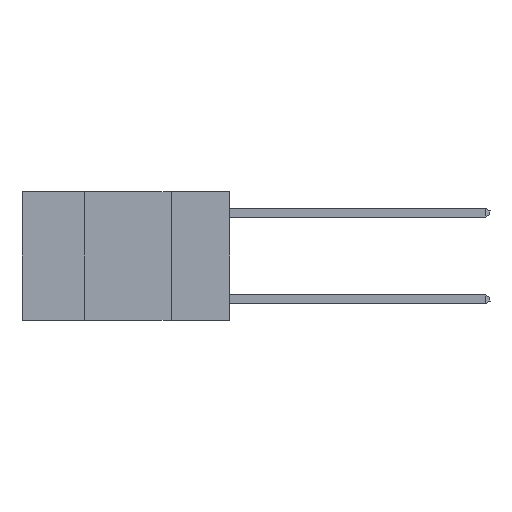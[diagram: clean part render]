
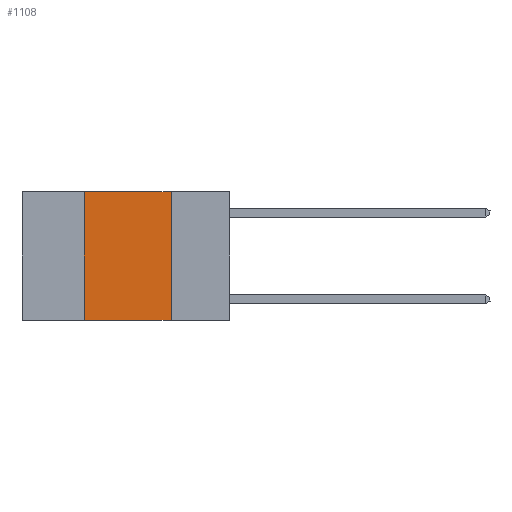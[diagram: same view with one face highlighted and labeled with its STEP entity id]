
A CAD part, left-side view. The second image highlights one B-rep face of the part: STEP entity #1108.
In plain terms, the highlighted planar face has unit normal (-1, 0, 0).
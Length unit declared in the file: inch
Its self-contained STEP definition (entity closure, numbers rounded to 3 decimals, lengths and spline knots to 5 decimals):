
#21 = CARTESIAN_POINT ( 'NONE',  ( 0., 0.17, 0. ) ) ;
#287 = LINE ( 'NONE', #9296, #6658 ) ;
#1108 = ADVANCED_FACE ( 'NONE', ( #13911 ), #3733, .F. ) ;
#1386 = ORIENTED_EDGE ( 'NONE', *, *, #11495, .F. ) ;
#1454 = EDGE_CURVE ( 'NONE', #6506, #8207, #287, .T. ) ;
#1458 = VERTEX_POINT ( 'NONE', #10606 ) ;
#2398 = CARTESIAN_POINT ( 'NONE',  ( 0., 0.17, 0. ) ) ;
#3000 = DIRECTION ( 'NONE',  ( 0., 0., 1. ) ) ;
#3733 = PLANE ( 'NONE',  #8202 ) ;
#3796 = ORIENTED_EDGE ( 'NONE', *, *, #1454, .T. ) ;
#3971 = VECTOR ( 'NONE', #3000, 39.37008 ) ;
#5261 = EDGE_CURVE ( 'NONE', #6506, #1458, #10196, .T. ) ;
#6243 = DIRECTION ( 'NONE',  ( 0., 0., -1. ) ) ;
#6506 = VERTEX_POINT ( 'NONE', #11076 ) ;
#6658 = VECTOR ( 'NONE', #8114, 39.37008 ) ;
#7731 = VECTOR ( 'NONE', #8714, 39.37008 ) ;
#7857 = EDGE_LOOP ( 'NONE', ( #13138, #1386, #8803, #3796 ) ) ;
#8114 = DIRECTION ( 'NONE',  ( 0., -1., 0. ) ) ;
#8202 = AXIS2_PLACEMENT_3D ( 'NONE', #9926, #13707, #6243 ) ;
#8207 = VERTEX_POINT ( 'NONE', #10542 ) ;
#8714 = DIRECTION ( 'NONE',  ( 0., -1., 0. ) ) ;
#8803 = ORIENTED_EDGE ( 'NONE', *, *, #5261, .F. ) ;
#9236 = LINE ( 'NONE', #21, #15153 ) ;
#9296 = CARTESIAN_POINT ( 'NONE',  ( 0., 0.6, -0.37 ) ) ;
#9926 = CARTESIAN_POINT ( 'NONE',  ( 0., 0.6, 0. ) ) ;
#10196 = LINE ( 'NONE', #11666, #3971 ) ;
#10542 = CARTESIAN_POINT ( 'NONE',  ( 0., 0.17, -0.37 ) ) ;
#10606 = CARTESIAN_POINT ( 'NONE',  ( 0., 0.42, 0. ) ) ;
#11076 = CARTESIAN_POINT ( 'NONE',  ( 0., 0.42, -0.37 ) ) ;
#11495 = EDGE_CURVE ( 'NONE', #1458, #12202, #14773, .T. ) ;
#11666 = CARTESIAN_POINT ( 'NONE',  ( 0., 0.42, 0. ) ) ;
#12202 = VERTEX_POINT ( 'NONE', #2398 ) ;
#12335 = EDGE_CURVE ( 'NONE', #12202, #8207, #9236, .T. ) ;
#13138 = ORIENTED_EDGE ( 'NONE', *, *, #12335, .F. ) ;
#13707 = DIRECTION ( 'NONE',  ( 1., 0., 0. ) ) ;
#13911 = FACE_OUTER_BOUND ( 'NONE', #7857, .T. ) ;
#14773 = LINE ( 'NONE', #14968, #7731 ) ;
#14968 = CARTESIAN_POINT ( 'NONE',  ( 0., 0.6, 0. ) ) ;
#15153 = VECTOR ( 'NONE', #15194, 39.37008 ) ;
#15194 = DIRECTION ( 'NONE',  ( 0., 0., -1. ) ) ;
